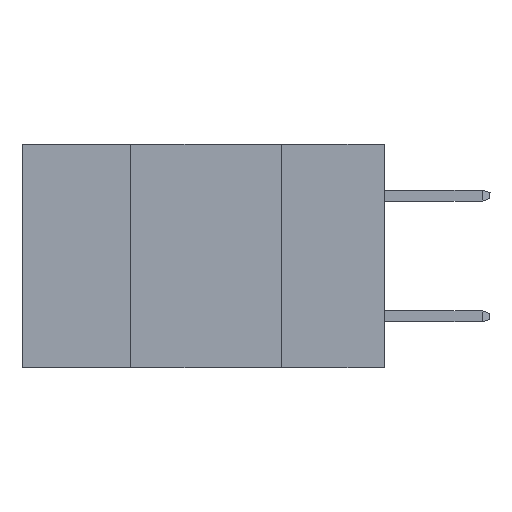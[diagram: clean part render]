
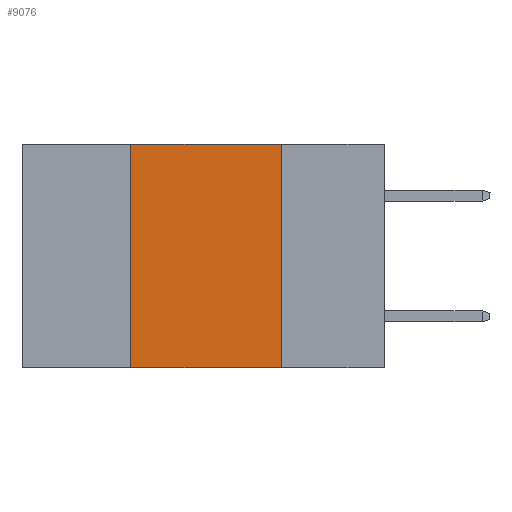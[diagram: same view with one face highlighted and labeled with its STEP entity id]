
A CAD part, left-side view. The second image highlights one B-rep face of the part: STEP entity #9076.
In plain terms, the highlighted planar face has unit normal (-1, 0, 0).
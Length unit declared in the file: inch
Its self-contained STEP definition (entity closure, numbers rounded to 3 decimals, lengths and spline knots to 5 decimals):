
#1002 = CARTESIAN_POINT ( 'NONE',  ( 0., 0.17, 0. ) ) ;
#2774 = EDGE_CURVE ( 'NONE', #6421, #12847, #7451, .T. ) ;
#3060 = EDGE_CURVE ( 'NONE', #6421, #4993, #5251, .T. ) ;
#3159 = CARTESIAN_POINT ( 'NONE',  ( 0., 0.17, -0.37 ) ) ;
#4274 = LINE ( 'NONE', #1002, #6957 ) ;
#4838 = DIRECTION ( 'NONE',  ( 0., -1., 0. ) ) ;
#4987 = EDGE_CURVE ( 'NONE', #4993, #8404, #5682, .T. ) ;
#4993 = VERTEX_POINT ( 'NONE', #10222 ) ;
#5142 = CARTESIAN_POINT ( 'NONE',  ( 0., 0.6, -0.37 ) ) ;
#5251 = LINE ( 'NONE', #5811, #7783 ) ;
#5635 = FACE_OUTER_BOUND ( 'NONE', #5771, .T. ) ;
#5682 = LINE ( 'NONE', #13133, #8399 ) ;
#5771 = EDGE_LOOP ( 'NONE', ( #7741, #6011, #11647, #11185 ) ) ;
#5811 = CARTESIAN_POINT ( 'NONE',  ( 0., 0.42, 0. ) ) ;
#6011 = ORIENTED_EDGE ( 'NONE', *, *, #4987, .F. ) ;
#6421 = VERTEX_POINT ( 'NONE', #9990 ) ;
#6957 = VECTOR ( 'NONE', #10806, 39.37008 ) ;
#7451 = LINE ( 'NONE', #5142, #13586 ) ;
#7741 = ORIENTED_EDGE ( 'NONE', *, *, #10521, .F. ) ;
#7783 = VECTOR ( 'NONE', #13455, 39.37008 ) ;
#8399 = VECTOR ( 'NONE', #4838, 39.37008 ) ;
#8404 = VERTEX_POINT ( 'NONE', #11728 ) ;
#8752 = CARTESIAN_POINT ( 'NONE',  ( 0., 0.6, 0. ) ) ;
#9076 = ADVANCED_FACE ( 'NONE', ( #5635 ), #11980, .F. ) ;
#9742 = DIRECTION ( 'NONE',  ( 1., 0., 0. ) ) ;
#9990 = CARTESIAN_POINT ( 'NONE',  ( 0., 0.42, -0.37 ) ) ;
#10222 = CARTESIAN_POINT ( 'NONE',  ( 0., 0.42, 0. ) ) ;
#10521 = EDGE_CURVE ( 'NONE', #8404, #12847, #4274, .T. ) ;
#10688 = DIRECTION ( 'NONE',  ( 0., 0., -1. ) ) ;
#10806 = DIRECTION ( 'NONE',  ( 0., 0., -1. ) ) ;
#11185 = ORIENTED_EDGE ( 'NONE', *, *, #2774, .T. ) ;
#11647 = ORIENTED_EDGE ( 'NONE', *, *, #3060, .F. ) ;
#11728 = CARTESIAN_POINT ( 'NONE',  ( 0., 0.17, 0. ) ) ;
#11980 = PLANE ( 'NONE',  #13910 ) ;
#12847 = VERTEX_POINT ( 'NONE', #3159 ) ;
#13133 = CARTESIAN_POINT ( 'NONE',  ( 0., 0.6, 0. ) ) ;
#13455 = DIRECTION ( 'NONE',  ( 0., 0., 1. ) ) ;
#13586 = VECTOR ( 'NONE', #13871, 39.37008 ) ;
#13871 = DIRECTION ( 'NONE',  ( 0., -1., 0. ) ) ;
#13910 = AXIS2_PLACEMENT_3D ( 'NONE', #8752, #9742, #10688 ) ;
